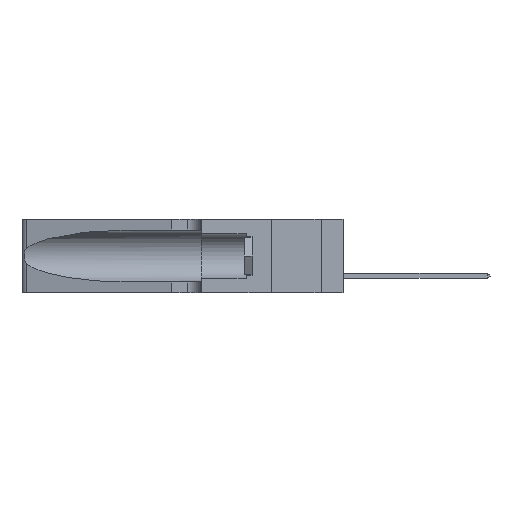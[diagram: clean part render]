
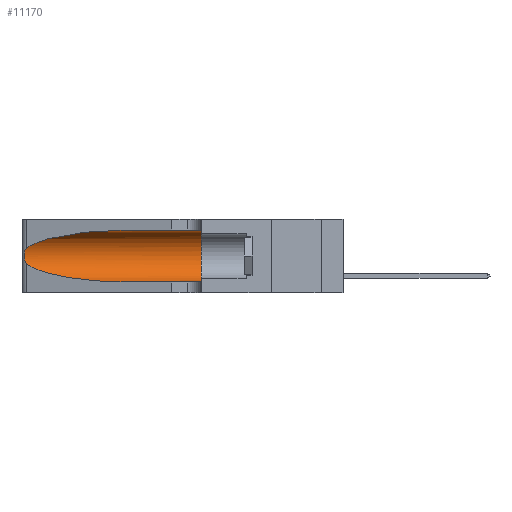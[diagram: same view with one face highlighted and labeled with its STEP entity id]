
A CAD part, left-side view. The second image highlights one B-rep face of the part: STEP entity #11170.
In plain terms, the highlighted cylindrical face has radius 3.308 mm (diameter 6.617 mm), a partial arc.
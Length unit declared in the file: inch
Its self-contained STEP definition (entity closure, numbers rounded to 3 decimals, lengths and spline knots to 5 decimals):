
#228 = DIRECTION ( 'NONE',  ( 0., -1., 0. ) ) ;
#605 = VERTEX_POINT ( 'NONE', #16454 ) ;
#839 = VERTEX_POINT ( 'NONE', #4178 ) ;
#868 = CARTESIAN_POINT ( 'NONE',  ( 0.25555, 1.22993, 0.14849 ) ) ;
#1152 = AXIS2_PLACEMENT_3D ( 'NONE', #12779, #12867, #7022 ) ;
#2399 = CARTESIAN_POINT ( 'NONE',  ( 0.1305, 0.72297, 0.05475 ) ) ;
#2453 = CARTESIAN_POINT ( 'NONE',  ( 0.25487, 1.22718, 0.22369 ) ) ;
#3866 = LINE ( 'NONE', #9741, #8922 ) ;
#4126 = CARTESIAN_POINT ( 'NONE',  ( 0.1305, 0.72297, 0.31525 ) ) ;
#4178 = CARTESIAN_POINT ( 'NONE',  ( 0.1305, 0.35, 0.31525 ) ) ;
#4384 = CARTESIAN_POINT ( 'NONE',  ( 0.25639, 1.23184, 0.21858 ) ) ;
#4387 = DIRECTION ( 'NONE',  ( 0., 0., 1. ) ) ;
#4464 = CARTESIAN_POINT ( 'NONE',  ( 0.26018, 1.23835, 0.19895 ) ) ;
#4499 = CARTESIAN_POINT ( 'NONE',  ( 0.18966, 0.96281, 0.05475 ) ) ;
#4721 = CARTESIAN_POINT ( 'NONE',  ( 0.25639, 1.23186, 0.15144 ) ) ;
#6307 = CARTESIAN_POINT ( 'NONE',  ( 0.26075, 1.23896, 0.178 ) ) ;
#6478 = CARTESIAN_POINT ( 'NONE',  ( 0.25555, 1.22994, 0.2215 ) ) ;
#6495 = EDGE_CURVE ( 'NONE', #15755, #9999, #11319, .T. ) ;
#7022 = DIRECTION ( 'NONE',  ( 0., 0., -1. ) ) ;
#7996 = ORIENTED_EDGE ( 'NONE', *, *, #10028, .F. ) ;
#8481 = CARTESIAN_POINT ( 'NONE',  ( 0.25856, 1.23593, 0.16098 ) ) ;
#8507 = EDGE_CURVE ( 'NONE', #16135, #605, #9442, .T. ) ;
#8922 = VECTOR ( 'NONE', #228, 39.37008 ) ;
#9442 = LINE ( 'NONE', #20930, #16585 ) ;
#9497 = EDGE_CURVE ( 'NONE', #9999, #16135, #23135, .T. ) ;
#9741 = CARTESIAN_POINT ( 'NONE',  ( 0.1305, 1.61858, 0.31525 ) ) ;
#9929 = CIRCLE ( 'NONE', #19157, 0.13025 ) ;
#9999 = VERTEX_POINT ( 'NONE', #12159 ) ;
#10028 = EDGE_CURVE ( 'NONE', #839, #605, #9929, .T. ) ;
#10093 = ORIENTED_EDGE ( 'NONE', *, *, #17576, .F. ) ;
#10317 = CARTESIAN_POINT ( 'NONE',  ( 0.25789, 1.23486, 0.15765 ) ) ;
#11170 = ADVANCED_FACE ( 'NONE', ( #17617 ), #15834, .F. ) ;
#11319 = B_SPLINE_CURVE_WITH_KNOTS ( 'NONE', 3,
 ( #2453, #6478, #4384, #21745, #19838, #4464, #14054, #6307, #17707, #8481, #10317, #4721, #868, #14209 ),
 .UNSPECIFIED., .F., .F.,
 ( 4, 2, 2, 2, 2, 2, 4 ),
 ( 0., 0.00027, 0.00053, 0.00107, 0.0016, 0.00187, 0.00214 ),
 .UNSPECIFIED. ) ;
#11783 = CARTESIAN_POINT ( 'NONE',  ( 0.25487, 1.22718, 0.14631 ) ) ;
#12017 = CARTESIAN_POINT ( 'NONE',  ( 0.1305, 0.72297, 0.31525 ) ) ;
#12080 = CARTESIAN_POINT ( 'NONE',  ( 0.1305, 0.35, 0.185 ) ) ;
#12159 = CARTESIAN_POINT ( 'NONE',  ( 0.25487, 1.22718, 0.14631 ) ) ;
#12779 = CARTESIAN_POINT ( 'NONE',  ( 0.1305, 1.61858, 0.185 ) ) ;
#12867 = DIRECTION ( 'NONE',  ( 0., -1., 0. ) ) ;
#13656 = CARTESIAN_POINT ( 'NONE',  ( 0.2373, 1.15595, 0.08982 ) ) ;
#14054 = CARTESIAN_POINT ( 'NONE',  ( 0.26075, 1.23896, 0.19203 ) ) ;
#14209 = CARTESIAN_POINT ( 'NONE',  ( 0.25487, 1.22718, 0.14631 ) ) ;
#14709 = ORIENTED_EDGE ( 'NONE', *, *, #8507, .T. ) ;
#15755 = VERTEX_POINT ( 'NONE', #17995 ) ;
#15804 = DIRECTION ( 'NONE',  ( 0., 1., 0. ) ) ;
#15829 = CARTESIAN_POINT ( 'NONE',  ( 0.2373, 1.15595, 0.28018 ) ) ;
#15834 = CYLINDRICAL_SURFACE ( 'NONE', #1152, 0.13025 ) ;
#16135 = VERTEX_POINT ( 'NONE', #16986 ) ;
#16386 = VERTEX_POINT ( 'NONE', #4126 ) ;
#16454 = CARTESIAN_POINT ( 'NONE',  ( 0.1305, 0.35, 0.05475 ) ) ;
#16585 = VECTOR ( 'NONE', #18931, 39.37008 ) ;
#16986 = CARTESIAN_POINT ( 'NONE',  ( 0.1305, 0.72297, 0.05475 ) ) ;
#17170 = EDGE_CURVE ( 'NONE', #16386, #15755, #20109, .T. ) ;
#17576 = EDGE_CURVE ( 'NONE', #16386, #839, #3866, .T. ) ;
#17617 = FACE_OUTER_BOUND ( 'NONE', #24190, .T. ) ;
#17707 = CARTESIAN_POINT ( 'NONE',  ( 0.26017, 1.23833, 0.17102 ) ) ;
#17739 = CARTESIAN_POINT ( 'NONE',  ( 0.25487, 1.22718, 0.22369 ) ) ;
#17995 = CARTESIAN_POINT ( 'NONE',  ( 0.25487, 1.22718, 0.22369 ) ) ;
#18931 = DIRECTION ( 'NONE',  ( 0., -1., 0. ) ) ;
#19157 = AXIS2_PLACEMENT_3D ( 'NONE', #12080, #15804, #4387 ) ;
#19368 = CARTESIAN_POINT ( 'NONE',  ( 0.18966, 0.96281, 0.31525 ) ) ;
#19838 = CARTESIAN_POINT ( 'NONE',  ( 0.25854, 1.2359, 0.20912 ) ) ;
#20109 =( BOUNDED_CURVE ( )  B_SPLINE_CURVE ( 3, ( #12017, #19368, #15829, #17739 ),
 .UNSPECIFIED., .F., .F. ) 
 B_SPLINE_CURVE_WITH_KNOTS ( ( 4, 4 ),
 ( 1.5708, 2.84003 ),
 .UNSPECIFIED. ) 
 CURVE ( )  GEOMETRIC_REPRESENTATION_ITEM ( )  RATIONAL_B_SPLINE_CURVE ( ( 1., 0.87, 0.87, 1. ) ) 
 REPRESENTATION_ITEM ( '' )  );
#20258 = ORIENTED_EDGE ( 'NONE', *, *, #9497, .T. ) ;
#20930 = CARTESIAN_POINT ( 'NONE',  ( 0.1305, 1.61858, 0.05475 ) ) ;
#21260 = ORIENTED_EDGE ( 'NONE', *, *, #17170, .T. ) ;
#21745 = CARTESIAN_POINT ( 'NONE',  ( 0.25787, 1.23484, 0.2124 ) ) ;
#23135 =( BOUNDED_CURVE ( )  B_SPLINE_CURVE ( 3, ( #11783, #13656, #4499, #2399 ),
 .UNSPECIFIED., .F., .T. ) 
 B_SPLINE_CURVE_WITH_KNOTS ( ( 4, 4 ),
 ( 3.44316, 4.71239 ),
 .UNSPECIFIED. ) 
 CURVE ( )  GEOMETRIC_REPRESENTATION_ITEM ( )  RATIONAL_B_SPLINE_CURVE ( ( 1., 0.87, 0.87, 1. ) ) 
 REPRESENTATION_ITEM ( '' )  );
#24190 = EDGE_LOOP ( 'NONE', ( #21260, #24548, #20258, #14709, #7996, #10093 ) ) ;
#24548 = ORIENTED_EDGE ( 'NONE', *, *, #6495, .T. ) ;
